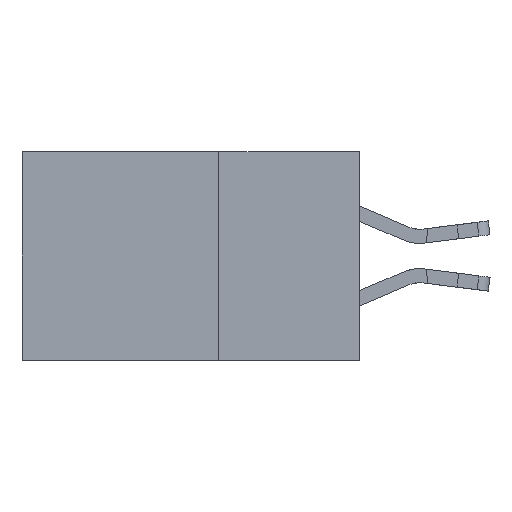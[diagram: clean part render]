
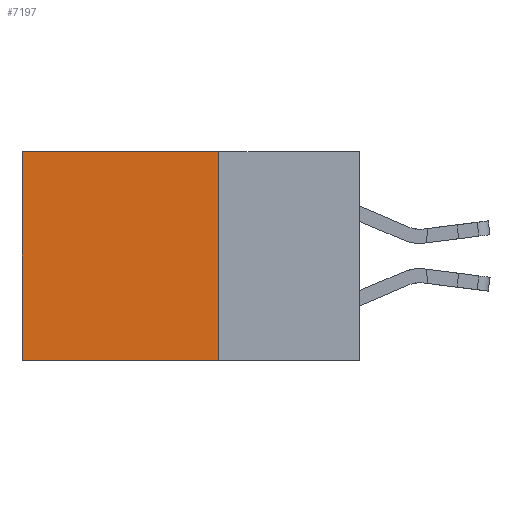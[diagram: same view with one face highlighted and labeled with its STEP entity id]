
A CAD part, left-side view. The second image highlights one B-rep face of the part: STEP entity #7197.
In plain terms, the highlighted planar face has unit normal (-1, 0, 0).
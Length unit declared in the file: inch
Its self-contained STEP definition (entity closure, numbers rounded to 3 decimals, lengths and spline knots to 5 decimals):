
#1321 = VERTEX_POINT ( 'NONE', #17482 ) ;
#1691 = ORIENTED_EDGE ( 'NONE', *, *, #6374, .F. ) ;
#1749 = VECTOR ( 'NONE', #5722, 39.37008 ) ;
#1934 = CARTESIAN_POINT ( 'NONE',  ( 0.2875, 0.25, 0. ) ) ;
#2809 = ORIENTED_EDGE ( 'NONE', *, *, #10623, .T. ) ;
#4136 = CARTESIAN_POINT ( 'NONE',  ( 0.2875, 0.6, 0. ) ) ;
#5469 = CARTESIAN_POINT ( 'NONE',  ( 0.2875, 0.25, -0.37 ) ) ;
#5722 = DIRECTION ( 'NONE',  ( 0., 0., -1. ) ) ;
#5933 = DIRECTION ( 'NONE',  ( 0., 1., 0. ) ) ;
#6374 = EDGE_CURVE ( 'NONE', #1321, #13938, #15822, .T. ) ;
#7026 = DIRECTION ( 'NONE',  ( 0., 1., 0. ) ) ;
#7029 = VERTEX_POINT ( 'NONE', #16152 ) ;
#7197 = ADVANCED_FACE ( 'NONE', ( #12607 ), #13440, .F. ) ;
#7214 = CARTESIAN_POINT ( 'NONE',  ( 0.2875, 0.25, 0. ) ) ;
#7840 = LINE ( 'NONE', #19919, #16153 ) ;
#7927 = VECTOR ( 'NONE', #7026, 39.37008 ) ;
#8669 = EDGE_CURVE ( 'NONE', #7029, #11859, #15730, .T. ) ;
#8767 = DIRECTION ( 'NONE',  ( 0., 0., -1. ) ) ;
#9881 = ORIENTED_EDGE ( 'NONE', *, *, #8669, .T. ) ;
#10048 = CARTESIAN_POINT ( 'NONE',  ( 0.2875, 0.6, -0.37 ) ) ;
#10623 = EDGE_CURVE ( 'NONE', #1321, #7029, #7840, .T. ) ;
#11620 = ORIENTED_EDGE ( 'NONE', *, *, #19153, .F. ) ;
#11650 = VECTOR ( 'NONE', #14472, 39.37008 ) ;
#11859 = VERTEX_POINT ( 'NONE', #10048 ) ;
#12607 = FACE_OUTER_BOUND ( 'NONE', #17030, .T. ) ;
#13440 = PLANE ( 'NONE',  #17501 ) ;
#13938 = VERTEX_POINT ( 'NONE', #13960 ) ;
#13960 = CARTESIAN_POINT ( 'NONE',  ( 0.2875, 0.25, -0.37 ) ) ;
#14472 = DIRECTION ( 'NONE',  ( 0., 0., -1. ) ) ;
#15730 = LINE ( 'NONE', #4136, #1749 ) ;
#15822 = LINE ( 'NONE', #1934, #11650 ) ;
#16152 = CARTESIAN_POINT ( 'NONE',  ( 0.2875, 0.6, 0. ) ) ;
#16153 = VECTOR ( 'NONE', #5933, 39.37008 ) ;
#16235 = LINE ( 'NONE', #5469, #7927 ) ;
#17030 = EDGE_LOOP ( 'NONE', ( #9881, #11620, #1691, #2809 ) ) ;
#17482 = CARTESIAN_POINT ( 'NONE',  ( 0.2875, 0.25, 0. ) ) ;
#17501 = AXIS2_PLACEMENT_3D ( 'NONE', #7214, #18093, #8767 ) ;
#18093 = DIRECTION ( 'NONE',  ( 1., 0., 0. ) ) ;
#19153 = EDGE_CURVE ( 'NONE', #13938, #11859, #16235, .T. ) ;
#19919 = CARTESIAN_POINT ( 'NONE',  ( 0.2875, 0.25, 0. ) ) ;
